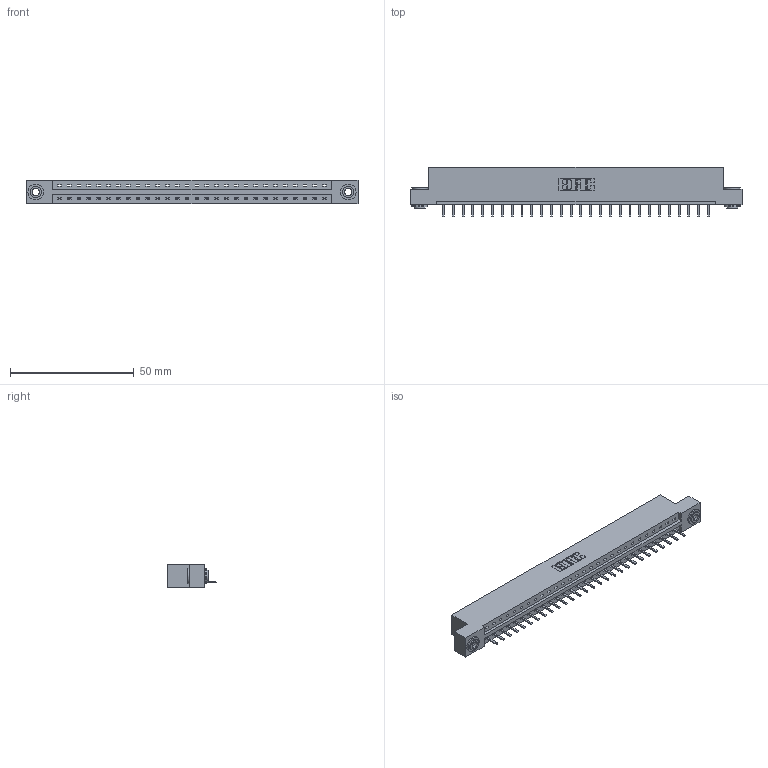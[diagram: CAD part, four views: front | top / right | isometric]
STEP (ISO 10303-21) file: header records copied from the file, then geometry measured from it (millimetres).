
FILE_DESCRIPTION (( 'STEP AP203' ), '1' );
FILE_NAME ('387-028-520-103.STEP', '2019-10-03T14:29:19', ( '' ), ( '' ), 'SwSTEP 2.0', 'SolidWorks 2016', '' );
FILE_SCHEMA (( 'CONFIG_CONTROL_DESIGN' ));
Length unit declared in the file: inch
Products named in the file (4): 345-292-001_345-293-120; 387-028-520-103; 337 Part_Flush Mounting Lugs - 0.156 Dia-TH; 345-250-002_345-250-002-102
Assembly tree (31 placements, depth 2):
  387-028-520-103
    337 Part_Flush Mounting Lugs - 0.156 Dia-TH
    345-292-001_345-293-120  x28
    345-250-002_345-250-002-102  x2
Bounding box: 133.96 x 20.02 x 9.4 mm (x, y, z)
Volume: 13686.5 mm3; surface area: 14008.1 mm2
Topology: 31 solids, 31 shells, 2000 faces, 5875 edges, 3838 vertices
Faces by surface type: plane 1424, cylinder 568, cone 8
Entity records: 23388 total; most frequent: CARTESIAN_POINT 4061, ORIENTED_EDGE 4006, DIRECTION 3469, EDGE_CURVE 2003, VECTOR 1847, LINE 1847, VERTEX_POINT 1330, AXIS2_PLACEMENT_3D 811
